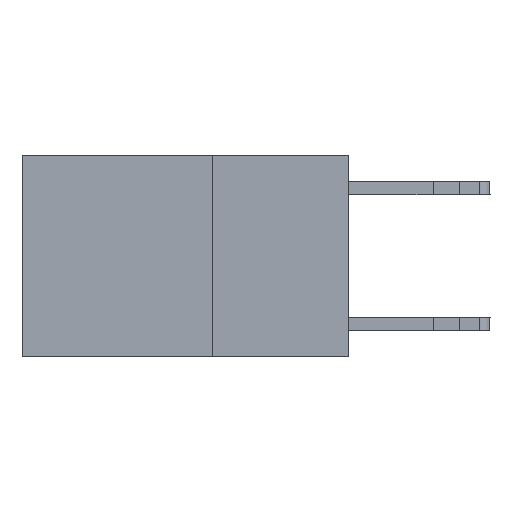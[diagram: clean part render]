
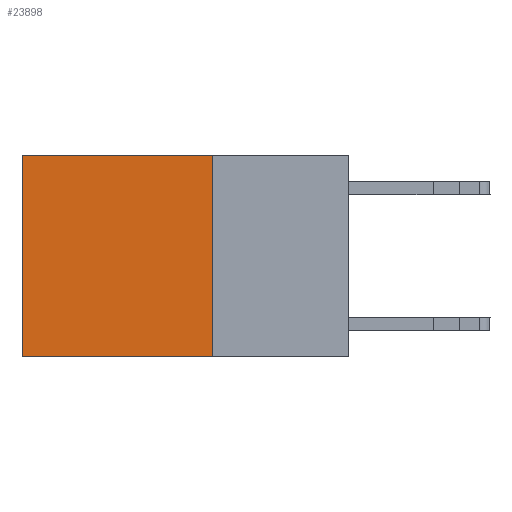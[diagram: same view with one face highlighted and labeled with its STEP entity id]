
A CAD part, left-side view. The second image highlights one B-rep face of the part: STEP entity #23898.
In plain terms, the highlighted planar face has unit normal (-1, 0, 0).
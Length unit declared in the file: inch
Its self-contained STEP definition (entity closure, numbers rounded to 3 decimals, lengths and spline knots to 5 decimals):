
#1711 = DIRECTION ( 'NONE',  ( 0., 0., -1. ) ) ;
#2686 = VECTOR ( 'NONE', #20765, 39.37008 ) ;
#3059 = ORIENTED_EDGE ( 'NONE', *, *, #16233, .F. ) ;
#3542 = CARTESIAN_POINT ( 'NONE',  ( 0.2625, 0.25, -0.37 ) ) ;
#4150 = CARTESIAN_POINT ( 'NONE',  ( 0.2625, 0.25, 0. ) ) ;
#4623 = ORIENTED_EDGE ( 'NONE', *, *, #24335, .F. ) ;
#6011 = VECTOR ( 'NONE', #25107, 39.37008 ) ;
#6314 = LINE ( 'NONE', #17195, #19962 ) ;
#8717 = EDGE_CURVE ( 'NONE', #18373, #13678, #6314, .T. ) ;
#9808 = FACE_OUTER_BOUND ( 'NONE', #15666, .T. ) ;
#10358 = VERTEX_POINT ( 'NONE', #3542 ) ;
#12205 = CARTESIAN_POINT ( 'NONE',  ( 0.2625, 0.25, -0.37 ) ) ;
#13045 = AXIS2_PLACEMENT_3D ( 'NONE', #25300, #16809, #18543 ) ;
#13515 = VECTOR ( 'NONE', #1711, 39.37008 ) ;
#13585 = EDGE_CURVE ( 'NONE', #27057, #18373, #16450, .T. ) ;
#13678 = VERTEX_POINT ( 'NONE', #24174 ) ;
#14913 = LINE ( 'NONE', #4150, #13515 ) ;
#15666 = EDGE_LOOP ( 'NONE', ( #23067, #3059, #4623, #19546 ) ) ;
#16233 = EDGE_CURVE ( 'NONE', #10358, #13678, #18494, .T. ) ;
#16248 = PLANE ( 'NONE',  #13045 ) ;
#16313 = CARTESIAN_POINT ( 'NONE',  ( 0.2625, 0.25, 0. ) ) ;
#16355 = CARTESIAN_POINT ( 'NONE',  ( 0.2625, 0.6, 0. ) ) ;
#16450 = LINE ( 'NONE', #16313, #2686 ) ;
#16809 = DIRECTION ( 'NONE',  ( 1., 0., 0. ) ) ;
#17195 = CARTESIAN_POINT ( 'NONE',  ( 0.2625, 0.6, 0. ) ) ;
#18373 = VERTEX_POINT ( 'NONE', #16355 ) ;
#18494 = LINE ( 'NONE', #12205, #6011 ) ;
#18543 = DIRECTION ( 'NONE',  ( 0., 0., -1. ) ) ;
#19546 = ORIENTED_EDGE ( 'NONE', *, *, #13585, .T. ) ;
#19962 = VECTOR ( 'NONE', #21390, 39.37008 ) ;
#20765 = DIRECTION ( 'NONE',  ( 0., 1., 0. ) ) ;
#21390 = DIRECTION ( 'NONE',  ( 0., 0., -1. ) ) ;
#23067 = ORIENTED_EDGE ( 'NONE', *, *, #8717, .T. ) ;
#23480 = CARTESIAN_POINT ( 'NONE',  ( 0.2625, 0.25, 0. ) ) ;
#23898 = ADVANCED_FACE ( 'NONE', ( #9808 ), #16248, .F. ) ;
#24174 = CARTESIAN_POINT ( 'NONE',  ( 0.2625, 0.6, -0.37 ) ) ;
#24335 = EDGE_CURVE ( 'NONE', #27057, #10358, #14913, .T. ) ;
#25107 = DIRECTION ( 'NONE',  ( 0., 1., 0. ) ) ;
#25300 = CARTESIAN_POINT ( 'NONE',  ( 0.2625, 0.25, 0. ) ) ;
#27057 = VERTEX_POINT ( 'NONE', #23480 ) ;
